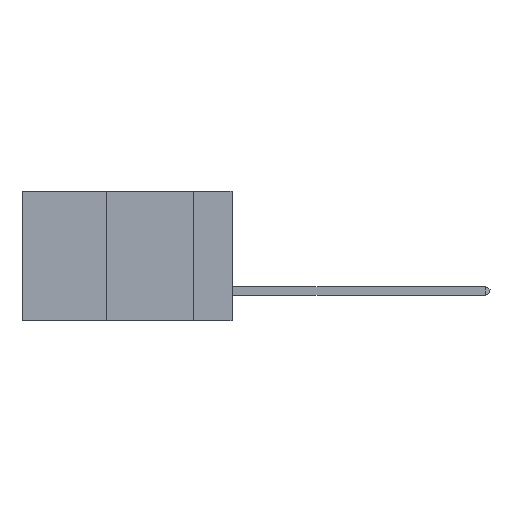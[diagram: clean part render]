
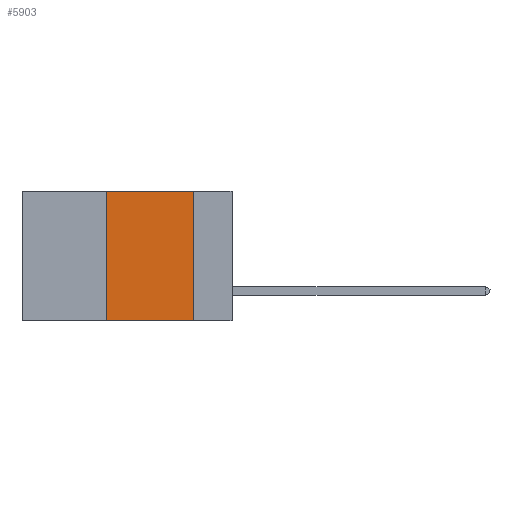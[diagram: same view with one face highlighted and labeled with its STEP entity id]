
A CAD part, left-side view. The second image highlights one B-rep face of the part: STEP entity #5903.
In plain terms, the highlighted planar face has unit normal (-1, 0, 0).
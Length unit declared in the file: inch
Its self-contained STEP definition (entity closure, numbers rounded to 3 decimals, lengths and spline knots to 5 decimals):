
#141 = DIRECTION ( 'NONE',  ( 0., -1., 0. ) ) ;
#215 = VERTEX_POINT ( 'NONE', #1704 ) ;
#268 = DIRECTION ( 'NONE',  ( 0., -1., 0. ) ) ;
#284 = CARTESIAN_POINT ( 'NONE',  ( 0., 0.11, 0. ) ) ;
#1606 = EDGE_CURVE ( 'NONE', #215, #4225, #6372, .T. ) ;
#1704 = CARTESIAN_POINT ( 'NONE',  ( 0., 0.36, -0.37 ) ) ;
#2695 = LINE ( 'NONE', #11748, #9053 ) ;
#2892 = VECTOR ( 'NONE', #8833, 39.37008 ) ;
#3453 = ORIENTED_EDGE ( 'NONE', *, *, #7592, .T. ) ;
#3662 = ORIENTED_EDGE ( 'NONE', *, *, #14761, .F. ) ;
#4225 = VERTEX_POINT ( 'NONE', #13463 ) ;
#4466 = PLANE ( 'NONE',  #9919 ) ;
#5903 = ADVANCED_FACE ( 'NONE', ( #16106 ), #4466, .F. ) ;
#5948 = ORIENTED_EDGE ( 'NONE', *, *, #1606, .F. ) ;
#6059 = CARTESIAN_POINT ( 'NONE',  ( 0., 0.36, 0. ) ) ;
#6372 = LINE ( 'NONE', #6059, #2892 ) ;
#6630 = EDGE_LOOP ( 'NONE', ( #14242, #3662, #5948, #3453 ) ) ;
#6753 = CARTESIAN_POINT ( 'NONE',  ( 0., 0.11, -0.37 ) ) ;
#6893 = VECTOR ( 'NONE', #268, 39.37008 ) ;
#7044 = CARTESIAN_POINT ( 'NONE',  ( 0., 0.6, 0. ) ) ;
#7165 = CARTESIAN_POINT ( 'NONE',  ( 0., 0.11, 0. ) ) ;
#7592 = EDGE_CURVE ( 'NONE', #215, #9509, #11382, .T. ) ;
#7850 = VERTEX_POINT ( 'NONE', #7165 ) ;
#8125 = CARTESIAN_POINT ( 'NONE',  ( 0., 0.6, -0.37 ) ) ;
#8578 = VECTOR ( 'NONE', #14874, 39.37008 ) ;
#8833 = DIRECTION ( 'NONE',  ( 0., 0., 1. ) ) ;
#9053 = VECTOR ( 'NONE', #141, 39.37008 ) ;
#9453 = DIRECTION ( 'NONE',  ( 1., 0., 0. ) ) ;
#9509 = VERTEX_POINT ( 'NONE', #6753 ) ;
#9919 = AXIS2_PLACEMENT_3D ( 'NONE', #7044, #9453, #10743 ) ;
#10743 = DIRECTION ( 'NONE',  ( 0., 0., -1. ) ) ;
#11310 = EDGE_CURVE ( 'NONE', #7850, #9509, #14840, .T. ) ;
#11382 = LINE ( 'NONE', #8125, #6893 ) ;
#11748 = CARTESIAN_POINT ( 'NONE',  ( 0., 0.6, 0. ) ) ;
#13463 = CARTESIAN_POINT ( 'NONE',  ( 0., 0.36, 0. ) ) ;
#14242 = ORIENTED_EDGE ( 'NONE', *, *, #11310, .F. ) ;
#14761 = EDGE_CURVE ( 'NONE', #4225, #7850, #2695, .T. ) ;
#14840 = LINE ( 'NONE', #284, #8578 ) ;
#14874 = DIRECTION ( 'NONE',  ( 0., 0., -1. ) ) ;
#16106 = FACE_OUTER_BOUND ( 'NONE', #6630, .T. ) ;
